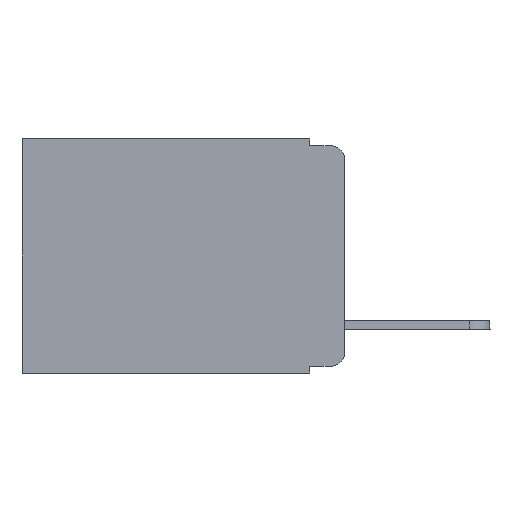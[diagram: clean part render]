
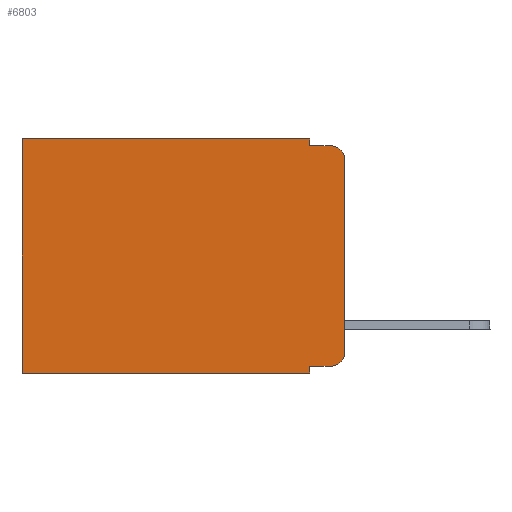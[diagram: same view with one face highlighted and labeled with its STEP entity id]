
A CAD part, left-side view. The second image highlights one B-rep face of the part: STEP entity #6803.
In plain terms, the highlighted planar face has unit normal (-1, 0, 0).
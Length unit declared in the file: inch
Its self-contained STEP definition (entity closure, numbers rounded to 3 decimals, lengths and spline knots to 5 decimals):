
#86 = DIRECTION ( 'NONE',  ( 0., 0., -1. ) ) ;
#902 = CARTESIAN_POINT ( 'NONE',  ( 0.298, 0., -0.343 ) ) ;
#965 = CARTESIAN_POINT ( 'NONE',  ( 0.298, 0.051, -0.333 ) ) ;
#1039 = EDGE_CURVE ( 'NONE', #4479, #11146, #13038, .T. ) ;
#1112 = CARTESIAN_POINT ( 'NONE',  ( 0.298, 0.473, 0. ) ) ;
#1143 = ORIENTED_EDGE ( 'NONE', *, *, #6155, .F. ) ;
#1237 = EDGE_CURVE ( 'NONE', #6878, #6444, #11177, .T. ) ;
#1514 = EDGE_CURVE ( 'NONE', #4479, #17507, #13381, .T. ) ;
#1670 = CARTESIAN_POINT ( 'NONE',  ( 0.298, 0., -0.03 ) ) ;
#1689 = LINE ( 'NONE', #16055, #1981 ) ;
#1981 = VECTOR ( 'NONE', #4448, 39.37008 ) ;
#2529 = DIRECTION ( 'NONE',  ( 1., 0., 0. ) ) ;
#2961 = CARTESIAN_POINT ( 'NONE',  ( 0.298, 0.051, 0. ) ) ;
#3452 = CIRCLE ( 'NONE', #14145, 0.02 ) ;
#3518 = ORIENTED_EDGE ( 'NONE', *, *, #1237, .F. ) ;
#3549 = EDGE_CURVE ( 'NONE', #11146, #13292, #3452, .T. ) ;
#3857 = CARTESIAN_POINT ( 'NONE',  ( 0.298, 0.051, -0.01 ) ) ;
#3903 = DIRECTION ( 'NONE',  ( 0., 0., -1. ) ) ;
#3959 = PLANE ( 'NONE',  #5927 ) ;
#4166 = VECTOR ( 'NONE', #11600, 39.37008 ) ;
#4448 = DIRECTION ( 'NONE',  ( 0., 0., -1. ) ) ;
#4479 = VERTEX_POINT ( 'NONE', #965 ) ;
#4793 = ORIENTED_EDGE ( 'NONE', *, *, #3549, .T. ) ;
#5094 = EDGE_CURVE ( 'NONE', #7695, #15593, #16465, .T. ) ;
#5407 = CARTESIAN_POINT ( 'NONE',  ( 0.298, 0.02, -0.01 ) ) ;
#5481 = DIRECTION ( 'NONE',  ( -1., 0., 0. ) ) ;
#5646 = ORIENTED_EDGE ( 'NONE', *, *, #8181, .F. ) ;
#5697 = VECTOR ( 'NONE', #13747, 39.37008 ) ;
#5763 = CARTESIAN_POINT ( 'NONE',  ( 0.298, 0.051, -0.333 ) ) ;
#5927 = AXIS2_PLACEMENT_3D ( 'NONE', #14025, #2529, #6743 ) ;
#6155 = EDGE_CURVE ( 'NONE', #7140, #13292, #8417, .T. ) ;
#6167 = EDGE_CURVE ( 'NONE', #15593, #14455, #14243, .T. ) ;
#6275 = CARTESIAN_POINT ( 'NONE',  ( 0.298, 0., -0.313 ) ) ;
#6444 = VERTEX_POINT ( 'NONE', #5407 ) ;
#6743 = DIRECTION ( 'NONE',  ( 0., 0., -1. ) ) ;
#6803 = ADVANCED_FACE ( 'NONE', ( #8188 ), #3959, .F. ) ;
#6878 = VERTEX_POINT ( 'NONE', #3857 ) ;
#7140 = VERTEX_POINT ( 'NONE', #1670 ) ;
#7543 = CARTESIAN_POINT ( 'NONE',  ( 0.298, 0.051, 0. ) ) ;
#7592 = EDGE_LOOP ( 'NONE', ( #1143, #8613, #3518, #13986, #14099, #18032, #5646, #17731, #18325, #4793 ) ) ;
#7695 = VERTEX_POINT ( 'NONE', #2961 ) ;
#8181 = EDGE_CURVE ( 'NONE', #17507, #14455, #15440, .T. ) ;
#8188 = FACE_OUTER_BOUND ( 'NONE', #7592, .T. ) ;
#8273 = CARTESIAN_POINT ( 'NONE',  ( 0.298, 0.02, -0.313 ) ) ;
#8328 = CARTESIAN_POINT ( 'NONE',  ( 0.298, 0.051, -0.01 ) ) ;
#8417 = LINE ( 'NONE', #17219, #15234 ) ;
#8527 = DIRECTION ( 'NONE',  ( 0., 0., -1. ) ) ;
#8613 = ORIENTED_EDGE ( 'NONE', *, *, #10642, .T. ) ;
#8894 = DIRECTION ( 'NONE',  ( -1., 0., 0. ) ) ;
#9097 = VECTOR ( 'NONE', #8527, 39.37008 ) ;
#9462 = CARTESIAN_POINT ( 'NONE',  ( 0.298, 0., 0. ) ) ;
#9929 = AXIS2_PLACEMENT_3D ( 'NONE', #14825, #8894, #86 ) ;
#10642 = EDGE_CURVE ( 'NONE', #7140, #6444, #18190, .T. ) ;
#10680 = CARTESIAN_POINT ( 'NONE',  ( 0.298, 0.02, -0.333 ) ) ;
#11016 = EDGE_CURVE ( 'NONE', #7695, #6878, #1689, .T. ) ;
#11146 = VERTEX_POINT ( 'NONE', #10680 ) ;
#11177 = LINE ( 'NONE', #8328, #18269 ) ;
#11600 = DIRECTION ( 'NONE',  ( 0., -1., 0. ) ) ;
#12659 = DIRECTION ( 'NONE',  ( 0., 0., -1. ) ) ;
#13038 = LINE ( 'NONE', #5763, #4166 ) ;
#13292 = VERTEX_POINT ( 'NONE', #6275 ) ;
#13381 = LINE ( 'NONE', #7543, #9097 ) ;
#13474 = CARTESIAN_POINT ( 'NONE',  ( 0.298, 0.473, -0.343 ) ) ;
#13504 = DIRECTION ( 'NONE',  ( 0., 1., 0. ) ) ;
#13747 = DIRECTION ( 'NONE',  ( 0., 1., 0. ) ) ;
#13986 = ORIENTED_EDGE ( 'NONE', *, *, #11016, .F. ) ;
#14025 = CARTESIAN_POINT ( 'NONE',  ( 0.298, 0., 0. ) ) ;
#14099 = ORIENTED_EDGE ( 'NONE', *, *, #5094, .T. ) ;
#14145 = AXIS2_PLACEMENT_3D ( 'NONE', #8273, #5481, #12659 ) ;
#14160 = VECTOR ( 'NONE', #13504, 39.37008 ) ;
#14243 = LINE ( 'NONE', #18735, #17627 ) ;
#14455 = VERTEX_POINT ( 'NONE', #13474 ) ;
#14825 = CARTESIAN_POINT ( 'NONE',  ( 0.298, 0.02, -0.03 ) ) ;
#15234 = VECTOR ( 'NONE', #18368, 39.37008 ) ;
#15440 = LINE ( 'NONE', #902, #5697 ) ;
#15593 = VERTEX_POINT ( 'NONE', #1112 ) ;
#16055 = CARTESIAN_POINT ( 'NONE',  ( 0.298, 0.051, 0. ) ) ;
#16465 = LINE ( 'NONE', #9462, #14160 ) ;
#17219 = CARTESIAN_POINT ( 'NONE',  ( 0.298, 0., 0. ) ) ;
#17507 = VERTEX_POINT ( 'NONE', #17708 ) ;
#17627 = VECTOR ( 'NONE', #3903, 39.37008 ) ;
#17708 = CARTESIAN_POINT ( 'NONE',  ( 0.298, 0.051, -0.343 ) ) ;
#17731 = ORIENTED_EDGE ( 'NONE', *, *, #1514, .F. ) ;
#18032 = ORIENTED_EDGE ( 'NONE', *, *, #6167, .T. ) ;
#18190 = CIRCLE ( 'NONE', #9929, 0.02 ) ;
#18269 = VECTOR ( 'NONE', #18375, 39.37008 ) ;
#18325 = ORIENTED_EDGE ( 'NONE', *, *, #1039, .T. ) ;
#18368 = DIRECTION ( 'NONE',  ( 0., 0., -1. ) ) ;
#18375 = DIRECTION ( 'NONE',  ( 0., -1., 0. ) ) ;
#18735 = CARTESIAN_POINT ( 'NONE',  ( 0.298, 0.473, 0. ) ) ;
